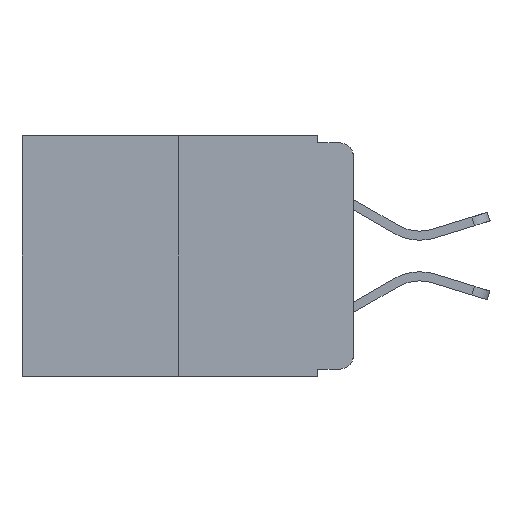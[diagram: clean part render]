
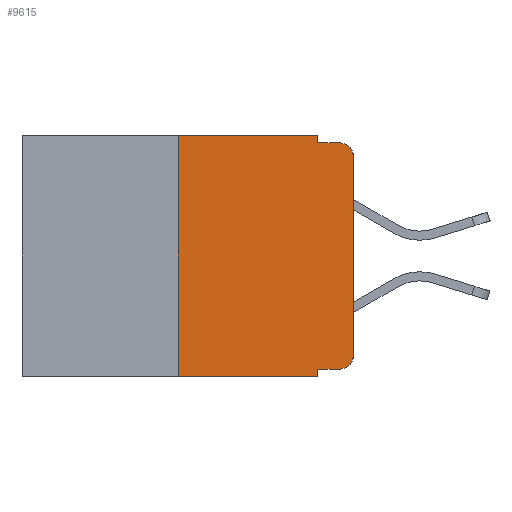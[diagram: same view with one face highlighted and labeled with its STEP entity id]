
A CAD part, left-side view. The second image highlights one B-rep face of the part: STEP entity #9615.
In plain terms, the highlighted planar face has unit normal (-1, 0, 0).
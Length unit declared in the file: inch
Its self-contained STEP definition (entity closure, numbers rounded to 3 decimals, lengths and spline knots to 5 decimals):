
#128 = CARTESIAN_POINT ( 'NONE',  ( 0., 0.473, 0. ) ) ;
#194 = DIRECTION ( 'NONE',  ( 0., 0., -1. ) ) ;
#457 = EDGE_CURVE ( 'NONE', #657, #15368, #10239, .T. ) ;
#536 = CARTESIAN_POINT ( 'NONE',  ( 0., 0.051, -0.01 ) ) ;
#636 = CARTESIAN_POINT ( 'NONE',  ( 0., 0., 0. ) ) ;
#657 = VERTEX_POINT ( 'NONE', #9783 ) ;
#776 = ORIENTED_EDGE ( 'NONE', *, *, #12818, .F. ) ;
#943 = CARTESIAN_POINT ( 'NONE',  ( 0., 0.051, -0.01 ) ) ;
#992 = CARTESIAN_POINT ( 'NONE',  ( 0., 0.473, -0.343 ) ) ;
#1216 = DIRECTION ( 'NONE',  ( 0., 0., -1. ) ) ;
#1326 = DIRECTION ( 'NONE',  ( 0., 0., 1. ) ) ;
#1337 = CARTESIAN_POINT ( 'NONE',  ( 0., 0.473, 0. ) ) ;
#2016 = DIRECTION ( 'NONE',  ( 0., -1., 0. ) ) ;
#2160 = VECTOR ( 'NONE', #3971, 39.37008 ) ;
#2351 = LINE ( 'NONE', #636, #12797 ) ;
#2557 = CARTESIAN_POINT ( 'NONE',  ( 0., 0.25, 0. ) ) ;
#2607 = LINE ( 'NONE', #1337, #9544 ) ;
#2815 = CARTESIAN_POINT ( 'NONE',  ( 0., 0.02, -0.313 ) ) ;
#3113 = VECTOR ( 'NONE', #7472, 39.37008 ) ;
#3229 = ORIENTED_EDGE ( 'NONE', *, *, #457, .T. ) ;
#3470 = VERTEX_POINT ( 'NONE', #12454 ) ;
#3526 = VERTEX_POINT ( 'NONE', #15966 ) ;
#3971 = DIRECTION ( 'NONE',  ( 0., 0., 1. ) ) ;
#4202 = ORIENTED_EDGE ( 'NONE', *, *, #4298, .T. ) ;
#4242 = DIRECTION ( 'NONE',  ( 0., 0., -1. ) ) ;
#4298 = EDGE_CURVE ( 'NONE', #3470, #657, #2351, .T. ) ;
#5051 = VERTEX_POINT ( 'NONE', #943 ) ;
#5059 = ORIENTED_EDGE ( 'NONE', *, *, #16266, .F. ) ;
#5364 = VERTEX_POINT ( 'NONE', #15111 ) ;
#5767 = VERTEX_POINT ( 'NONE', #15746 ) ;
#5892 = VERTEX_POINT ( 'NONE', #14727 ) ;
#6060 = CARTESIAN_POINT ( 'NONE',  ( 0., 0.051, -0.333 ) ) ;
#6138 = ORIENTED_EDGE ( 'NONE', *, *, #17115, .F. ) ;
#6182 = ORIENTED_EDGE ( 'NONE', *, *, #6977, .T. ) ;
#6558 = EDGE_LOOP ( 'NONE', ( #4202, #3229, #6138, #5059, #776, #12708, #6182, #7423, #8011, #11562 ) ) ;
#6668 = FACE_OUTER_BOUND ( 'NONE', #6558, .T. ) ;
#6731 = AXIS2_PLACEMENT_3D ( 'NONE', #2815, #12368, #4242 ) ;
#6791 = LINE ( 'NONE', #14892, #10830 ) ;
#6977 = EDGE_CURVE ( 'NONE', #5892, #3526, #16571, .T. ) ;
#7252 = PLANE ( 'NONE',  #11800 ) ;
#7256 = LINE ( 'NONE', #6060, #3113 ) ;
#7423 = ORIENTED_EDGE ( 'NONE', *, *, #14529, .F. ) ;
#7472 = DIRECTION ( 'NONE',  ( 0., -1., 0. ) ) ;
#7923 = LINE ( 'NONE', #536, #14512 ) ;
#8011 = ORIENTED_EDGE ( 'NONE', *, *, #13665, .T. ) ;
#8321 = DIRECTION ( 'NONE',  ( 0., -1., 0. ) ) ;
#8621 = DIRECTION ( 'NONE',  ( 1., 0., 0. ) ) ;
#8658 = DIRECTION ( 'NONE',  ( 0., 0., -1. ) ) ;
#9220 = VECTOR ( 'NONE', #15925, 39.37008 ) ;
#9544 = VECTOR ( 'NONE', #8321, 39.37008 ) ;
#9615 = ADVANCED_FACE ( 'NONE', ( #6668 ), #7252, .F. ) ;
#9783 = CARTESIAN_POINT ( 'NONE',  ( 0., 0., -0.03 ) ) ;
#10239 = CIRCLE ( 'NONE', #13397, 0.02 ) ;
#10455 = CIRCLE ( 'NONE', #6731, 0.02 ) ;
#10830 = VECTOR ( 'NONE', #1216, 39.37008 ) ;
#11045 = EDGE_CURVE ( 'NONE', #5364, #3470, #10455, .T. ) ;
#11303 = CARTESIAN_POINT ( 'NONE',  ( 0., 0.051, 0. ) ) ;
#11331 = CARTESIAN_POINT ( 'NONE',  ( 0., 0.02, -0.03 ) ) ;
#11562 = ORIENTED_EDGE ( 'NONE', *, *, #11045, .T. ) ;
#11784 = VECTOR ( 'NONE', #8658, 39.37008 ) ;
#11800 = AXIS2_PLACEMENT_3D ( 'NONE', #128, #8621, #194 ) ;
#12028 = CARTESIAN_POINT ( 'NONE',  ( 0., 0.02, -0.01 ) ) ;
#12090 = VERTEX_POINT ( 'NONE', #15781 ) ;
#12368 = DIRECTION ( 'NONE',  ( -1., 0., 0. ) ) ;
#12454 = CARTESIAN_POINT ( 'NONE',  ( 0., 0., -0.313 ) ) ;
#12708 = ORIENTED_EDGE ( 'NONE', *, *, #15398, .F. ) ;
#12797 = VECTOR ( 'NONE', #1326, 39.37008 ) ;
#12818 = EDGE_CURVE ( 'NONE', #15359, #12090, #2607, .T. ) ;
#13030 = LINE ( 'NONE', #2557, #2160 ) ;
#13397 = AXIS2_PLACEMENT_3D ( 'NONE', #11331, #13846, #13878 ) ;
#13665 = EDGE_CURVE ( 'NONE', #5767, #5364, #7256, .T. ) ;
#13846 = DIRECTION ( 'NONE',  ( -1., 0., 0. ) ) ;
#13878 = DIRECTION ( 'NONE',  ( 0., 0., -1. ) ) ;
#14512 = VECTOR ( 'NONE', #2016, 39.37008 ) ;
#14529 = EDGE_CURVE ( 'NONE', #5767, #3526, #6791, .T. ) ;
#14614 = CARTESIAN_POINT ( 'NONE',  ( 0., 0.25, 0. ) ) ;
#14727 = CARTESIAN_POINT ( 'NONE',  ( 0., 0.25, -0.343 ) ) ;
#14892 = CARTESIAN_POINT ( 'NONE',  ( 0., 0.051, 0. ) ) ;
#15111 = CARTESIAN_POINT ( 'NONE',  ( 0., 0.02, -0.333 ) ) ;
#15215 = LINE ( 'NONE', #11303, #11784 ) ;
#15359 = VERTEX_POINT ( 'NONE', #14614 ) ;
#15368 = VERTEX_POINT ( 'NONE', #12028 ) ;
#15398 = EDGE_CURVE ( 'NONE', #5892, #15359, #13030, .T. ) ;
#15746 = CARTESIAN_POINT ( 'NONE',  ( 0., 0.051, -0.333 ) ) ;
#15781 = CARTESIAN_POINT ( 'NONE',  ( 0., 0.051, 0. ) ) ;
#15925 = DIRECTION ( 'NONE',  ( 0., -1., 0. ) ) ;
#15966 = CARTESIAN_POINT ( 'NONE',  ( 0., 0.051, -0.343 ) ) ;
#16266 = EDGE_CURVE ( 'NONE', #12090, #5051, #15215, .T. ) ;
#16571 = LINE ( 'NONE', #992, #9220 ) ;
#17115 = EDGE_CURVE ( 'NONE', #5051, #15368, #7923, .T. ) ;
